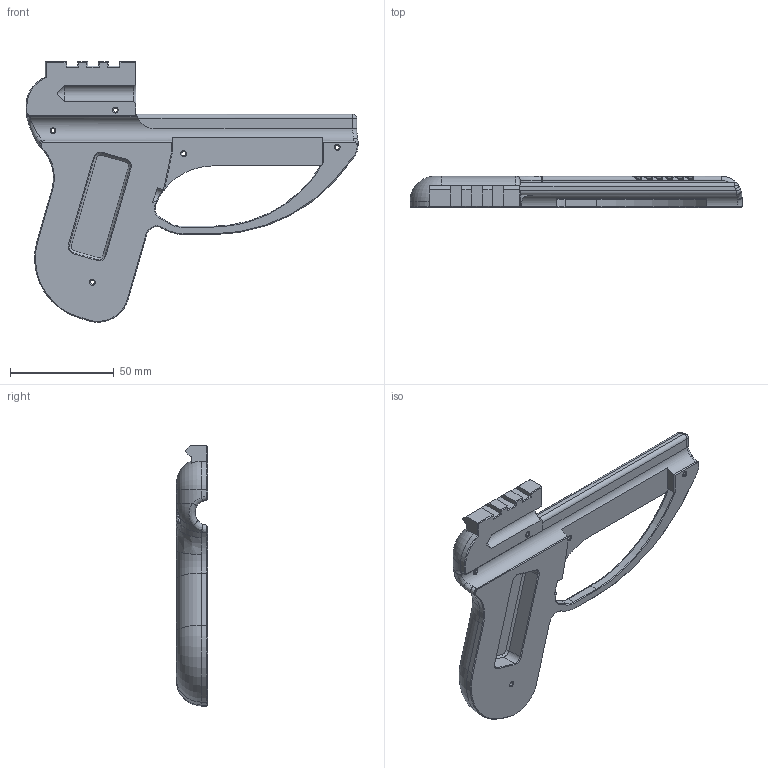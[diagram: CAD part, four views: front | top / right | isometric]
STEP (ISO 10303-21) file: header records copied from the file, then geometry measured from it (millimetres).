
FILE_DESCRIPTION(('FreeCAD Model'),'2;1');
FILE_NAME('Open CASCADE Shape Model','2022-12-07T11:24:18',('Author'),( ''),'Open CASCADE STEP processor 7.6','FreeCAD','Unknown');
FILE_SCHEMA(('AUTOMOTIVE_DESIGN { 1 0 10303 214 1 1 1 1 }'));
Length unit declared in the file: millimetre
Products named in the file (1): Frame-Left-Pic
Bounding box: 160 x 15 x 125.44 mm (x, y, z)
Volume: 90760 mm3; surface area: 26802.4 mm2
Topology: 1 solids, 1 shells, 696 faces, 1877 edges, 1181 vertices
Faces by surface type: plane 420, bspline 154, cylinder 70, cone 32, torus 16, revolution 4
Full cylindrical faces by diameter (mm): 2 x5
Entity records: 64951 total; most frequent: CARTESIAN_POINT 31406, DIRECTION 5003, ORIENTED_EDGE 3748, PCURVE 3748, DEFINITIONAL_REPRESENTATION 3748, LINE 3520, VECTOR 3520, EDGE_CURVE 1874
